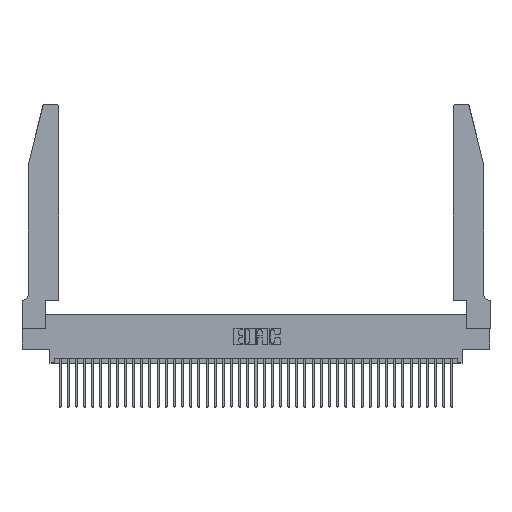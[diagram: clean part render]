
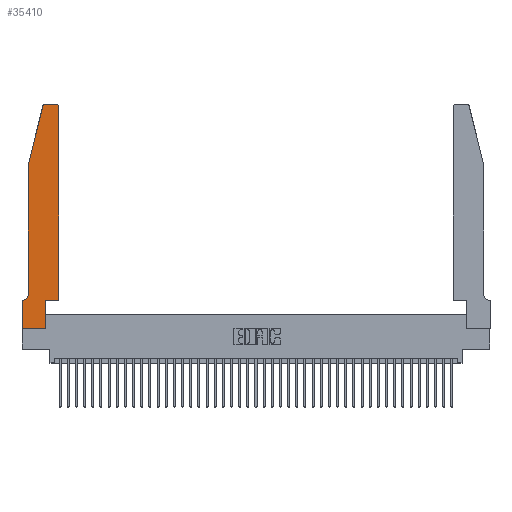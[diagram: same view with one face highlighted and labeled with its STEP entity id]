
A CAD part, top view. The second image highlights one B-rep face of the part: STEP entity #35410.
In plain terms, the highlighted planar face has unit normal (0, 0, 1).
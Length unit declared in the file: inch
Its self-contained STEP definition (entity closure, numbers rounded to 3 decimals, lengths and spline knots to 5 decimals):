
#112 = EDGE_CURVE ( 'NONE', #20316, #9884, #13374, .T. ) ;
#523 = EDGE_CURVE ( 'NONE', #9884, #19165, #28243, .T. ) ;
#626 = AXIS2_PLACEMENT_3D ( 'NONE', #789, #4381, #1231 ) ;
#789 = CARTESIAN_POINT ( 'NONE',  ( 0., 0.35, 0.37 ) ) ;
#926 = EDGE_CURVE ( 'NONE', #10603, #31893, #38432, .T. ) ;
#960 = DIRECTION ( 'NONE',  ( -1., 0., 0. ) ) ;
#1231 = DIRECTION ( 'NONE',  ( 1., 0., 0. ) ) ;
#1753 = EDGE_CURVE ( 'NONE', #41255, #17285, #40989, .T. ) ;
#1940 = CARTESIAN_POINT ( 'NONE',  ( 0.4205, 2.72, 0.37 ) ) ;
#2105 = DIRECTION ( 'NONE',  ( 0., 0., 1. ) ) ;
#3840 = FACE_OUTER_BOUND ( 'NONE', #39535, .T. ) ;
#4381 = DIRECTION ( 'NONE',  ( 0., 0., 1. ) ) ;
#5065 = VECTOR ( 'NONE', #6164, 39.37008 ) ;
#5259 = CARTESIAN_POINT ( 'NONE',  ( 0.4505, 0.35, 0.37 ) ) ;
#5572 = CARTESIAN_POINT ( 'NONE',  ( 0.0055, 0.35, 0.37 ) ) ;
#5954 = DIRECTION ( 'NONE',  ( 0., 0., -1. ) ) ;
#6164 = DIRECTION ( 'NONE',  ( -1., 0., 0. ) ) ;
#6741 = EDGE_CURVE ( 'NONE', #23564, #10299, #10150, .T. ) ;
#6906 = CARTESIAN_POINT ( 'NONE',  ( 0.2865, 0., 0.37 ) ) ;
#7397 = EDGE_CURVE ( 'NONE', #36206, #10603, #37799, .T. ) ;
#9473 = VECTOR ( 'NONE', #10115, 39.37008 ) ;
#9749 = CARTESIAN_POINT ( 'NONE',  ( 0.4205, 2.75, 0.37 ) ) ;
#9884 = VERTEX_POINT ( 'NONE', #27712 ) ;
#10115 = DIRECTION ( 'NONE',  ( -0.239, -0.971, 0. ) ) ;
#10150 = LINE ( 'NONE', #26816, #27585 ) ;
#10299 = VERTEX_POINT ( 'NONE', #32429 ) ;
#10406 = CARTESIAN_POINT ( 'NONE',  ( 0.284, 2.75, 0.37 ) ) ;
#10603 = VERTEX_POINT ( 'NONE', #23935 ) ;
#10774 = AXIS2_PLACEMENT_3D ( 'NONE', #11539, #2105, #34561 ) ;
#11215 = VERTEX_POINT ( 'NONE', #14210 ) ;
#11342 = CARTESIAN_POINT ( 'NONE',  ( 0.4505, 2.72, 0.37 ) ) ;
#11539 = CARTESIAN_POINT ( 'NONE',  ( 0.284, 2.72, 0.37 ) ) ;
#12013 = CARTESIAN_POINT ( 'NONE',  ( 0.2605, 2.75, 0.37 ) ) ;
#12854 = ORIENTED_EDGE ( 'NONE', *, *, #6741, .T. ) ;
#13077 = CARTESIAN_POINT ( 'NONE',  ( 0., 0., 0.37 ) ) ;
#13374 = LINE ( 'NONE', #40519, #15905 ) ;
#13638 = DIRECTION ( 'NONE',  ( -1., 0., 0. ) ) ;
#14201 = AXIS2_PLACEMENT_3D ( 'NONE', #22281, #5954, #13638 ) ;
#14210 = CARTESIAN_POINT ( 'NONE',  ( 0.25487, 2.72718, 0.37 ) ) ;
#14304 = EDGE_CURVE ( 'NONE', #17285, #11215, #30456, .T. ) ;
#15265 = EDGE_CURVE ( 'NONE', #31893, #21505, #29828, .T. ) ;
#15445 = VECTOR ( 'NONE', #29083, 39.37008 ) ;
#15905 = VECTOR ( 'NONE', #960, 39.37008 ) ;
#17207 = ORIENTED_EDGE ( 'NONE', *, *, #15265, .T. ) ;
#17285 = VERTEX_POINT ( 'NONE', #10406 ) ;
#18017 = EDGE_CURVE ( 'NONE', #21505, #41255, #31039, .T. ) ;
#18458 = VECTOR ( 'NONE', #33516, 39.37008 ) ;
#18778 = EDGE_CURVE ( 'NONE', #11215, #23564, #25335, .T. ) ;
#19028 = LINE ( 'NONE', #20119, #41130 ) ;
#19165 = VERTEX_POINT ( 'NONE', #37414 ) ;
#19347 = VECTOR ( 'NONE', #41675, 39.37008 ) ;
#20119 = CARTESIAN_POINT ( 'NONE',  ( 0., 0., 0.37 ) ) ;
#20316 = VERTEX_POINT ( 'NONE', #5572 ) ;
#20550 = DIRECTION ( 'NONE',  ( 0., -1., 0. ) ) ;
#21505 = VERTEX_POINT ( 'NONE', #11342 ) ;
#21900 = EDGE_CURVE ( 'NONE', #10299, #20316, #30187, .T. ) ;
#22281 = CARTESIAN_POINT ( 'NONE',  ( 0.0055, 0.42, 0.37 ) ) ;
#22626 = DIRECTION ( 'NONE',  ( 1., 0., 0. ) ) ;
#22851 = ORIENTED_EDGE ( 'NONE', *, *, #18017, .T. ) ;
#23248 = DIRECTION ( 'NONE',  ( 1., 0., 0. ) ) ;
#23563 = PLANE ( 'NONE',  #626 ) ;
#23564 = VERTEX_POINT ( 'NONE', #34999 ) ;
#23935 = CARTESIAN_POINT ( 'NONE',  ( 0.2865, 0.35, 0.37 ) ) ;
#25335 = LINE ( 'NONE', #32459, #9473 ) ;
#25392 = AXIS2_PLACEMENT_3D ( 'NONE', #1940, #31394, #41337 ) ;
#25654 = EDGE_CURVE ( 'NONE', #19165, #36206, #19028, .T. ) ;
#26816 = CARTESIAN_POINT ( 'NONE',  ( 0.0755, 2., 0.37 ) ) ;
#27585 = VECTOR ( 'NONE', #20550, 39.37008 ) ;
#27712 = CARTESIAN_POINT ( 'NONE',  ( 0., 0.35, 0.37 ) ) ;
#27728 = ORIENTED_EDGE ( 'NONE', *, *, #523, .T. ) ;
#28206 = VECTOR ( 'NONE', #22626, 39.37008 ) ;
#28243 = LINE ( 'NONE', #13077, #18458 ) ;
#28384 = ORIENTED_EDGE ( 'NONE', *, *, #112, .T. ) ;
#28457 = CARTESIAN_POINT ( 'NONE',  ( 0.2865, 0.35, 0.37 ) ) ;
#28857 = ORIENTED_EDGE ( 'NONE', *, *, #7397, .T. ) ;
#29083 = DIRECTION ( 'NONE',  ( 0., 1., 0. ) ) ;
#29828 = LINE ( 'NONE', #35184, #15445 ) ;
#30187 = CIRCLE ( 'NONE', #14201, 0.07 ) ;
#30456 = CIRCLE ( 'NONE', #10774, 0.03 ) ;
#30763 = ORIENTED_EDGE ( 'NONE', *, *, #25654, .T. ) ;
#31039 = CIRCLE ( 'NONE', #25392, 0.03 ) ;
#31394 = DIRECTION ( 'NONE',  ( 0., 0., 1. ) ) ;
#31893 = VERTEX_POINT ( 'NONE', #5259 ) ;
#32429 = CARTESIAN_POINT ( 'NONE',  ( 0.0755, 0.42, 0.37 ) ) ;
#32459 = CARTESIAN_POINT ( 'NONE',  ( 0.0755, 2., 0.37 ) ) ;
#32742 = ORIENTED_EDGE ( 'NONE', *, *, #21900, .T. ) ;
#33516 = DIRECTION ( 'NONE',  ( 0., -1., 0. ) ) ;
#34561 = DIRECTION ( 'NONE',  ( 1., 0., 0. ) ) ;
#34999 = CARTESIAN_POINT ( 'NONE',  ( 0.0755, 2., 0.37 ) ) ;
#35184 = CARTESIAN_POINT ( 'NONE',  ( 0.4505, 0.35, 0.37 ) ) ;
#35410 = ADVANCED_FACE ( 'NONE', ( #3840 ), #23563, .T. ) ;
#35419 = ORIENTED_EDGE ( 'NONE', *, *, #18778, .T. ) ;
#35611 = CARTESIAN_POINT ( 'NONE',  ( 0.4505, 0.35, 0.37 ) ) ;
#36206 = VERTEX_POINT ( 'NONE', #6906 ) ;
#37125 = ORIENTED_EDGE ( 'NONE', *, *, #14304, .T. ) ;
#37414 = CARTESIAN_POINT ( 'NONE',  ( 0., 0., 0.37 ) ) ;
#37799 = LINE ( 'NONE', #28457, #19347 ) ;
#38432 = LINE ( 'NONE', #35611, #28206 ) ;
#39535 = EDGE_LOOP ( 'NONE', ( #41836, #37125, #35419, #12854, #32742, #28384, #27728, #30763, #28857, #40042, #17207, #22851 ) ) ;
#40042 = ORIENTED_EDGE ( 'NONE', *, *, #926, .T. ) ;
#40519 = CARTESIAN_POINT ( 'NONE',  ( 0.0755, 0.35, 0.37 ) ) ;
#40989 = LINE ( 'NONE', #12013, #5065 ) ;
#41130 = VECTOR ( 'NONE', #23248, 39.37008 ) ;
#41255 = VERTEX_POINT ( 'NONE', #9749 ) ;
#41337 = DIRECTION ( 'NONE',  ( 1., 0., 0. ) ) ;
#41675 = DIRECTION ( 'NONE',  ( 0., 1., 0. ) ) ;
#41836 = ORIENTED_EDGE ( 'NONE', *, *, #1753, .T. ) ;
